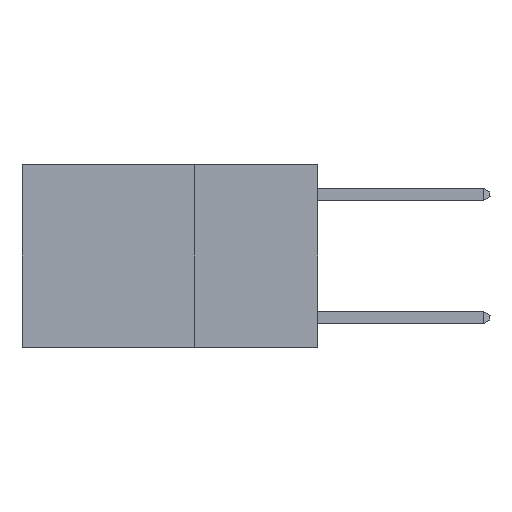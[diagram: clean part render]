
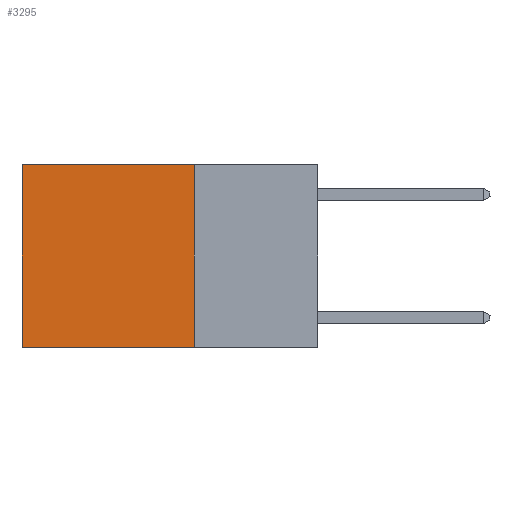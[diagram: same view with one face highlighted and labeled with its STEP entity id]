
A CAD part, left-side view. The second image highlights one B-rep face of the part: STEP entity #3295.
In plain terms, the highlighted planar face has unit normal (-1, 0, 0).
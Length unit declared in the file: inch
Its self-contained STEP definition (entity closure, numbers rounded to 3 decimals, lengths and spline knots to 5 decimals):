
#916 = ORIENTED_EDGE ( 'NONE', *, *, #24766, .T. ) ;
#2970 = VECTOR ( 'NONE', #10923, 39.37008 ) ;
#3295 = ADVANCED_FACE ( 'NONE', ( #18568 ), #12385, .F. ) ;
#3473 = DIRECTION ( 'NONE',  ( 1., 0., 0. ) ) ;
#4056 = DIRECTION ( 'NONE',  ( 0., 0., -1. ) ) ;
#4221 = VERTEX_POINT ( 'NONE', #8551 ) ;
#4352 = VERTEX_POINT ( 'NONE', #13486 ) ;
#6015 = ORIENTED_EDGE ( 'NONE', *, *, #16550, .F. ) ;
#8277 = CARTESIAN_POINT ( 'NONE',  ( 0.2625, 0.6, 0. ) ) ;
#8551 = CARTESIAN_POINT ( 'NONE',  ( 0.2625, 0.6, -0.37 ) ) ;
#8670 = CARTESIAN_POINT ( 'NONE',  ( 0.2625, 0.25, -0.37 ) ) ;
#10423 = LINE ( 'NONE', #16756, #11601 ) ;
#10604 = ORIENTED_EDGE ( 'NONE', *, *, #14463, .T. ) ;
#10695 = VECTOR ( 'NONE', #12228, 39.37008 ) ;
#10923 = DIRECTION ( 'NONE',  ( 0., 1., 0. ) ) ;
#11601 = VECTOR ( 'NONE', #4056, 39.37008 ) ;
#12228 = DIRECTION ( 'NONE',  ( 0., 0., -1. ) ) ;
#12278 = CARTESIAN_POINT ( 'NONE',  ( 0.2625, 0.25, 0. ) ) ;
#12385 = PLANE ( 'NONE',  #26535 ) ;
#12756 = VERTEX_POINT ( 'NONE', #12278 ) ;
#13092 = EDGE_LOOP ( 'NONE', ( #916, #6015, #21237, #10604 ) ) ;
#13486 = CARTESIAN_POINT ( 'NONE',  ( 0.2625, 0.25, -0.37 ) ) ;
#14463 = EDGE_CURVE ( 'NONE', #12756, #21655, #22265, .T. ) ;
#16550 = EDGE_CURVE ( 'NONE', #4352, #4221, #27836, .T. ) ;
#16756 = CARTESIAN_POINT ( 'NONE',  ( 0.2625, 0.25, 0. ) ) ;
#16844 = LINE ( 'NONE', #23070, #10695 ) ;
#17930 = EDGE_CURVE ( 'NONE', #12756, #4352, #10423, .T. ) ;
#18568 = FACE_OUTER_BOUND ( 'NONE', #13092, .T. ) ;
#20975 = DIRECTION ( 'NONE',  ( 0., 0., -1. ) ) ;
#21237 = ORIENTED_EDGE ( 'NONE', *, *, #17930, .F. ) ;
#21655 = VERTEX_POINT ( 'NONE', #8277 ) ;
#22265 = LINE ( 'NONE', #24377, #25045 ) ;
#23070 = CARTESIAN_POINT ( 'NONE',  ( 0.2625, 0.6, 0. ) ) ;
#24377 = CARTESIAN_POINT ( 'NONE',  ( 0.2625, 0.25, 0. ) ) ;
#24766 = EDGE_CURVE ( 'NONE', #21655, #4221, #16844, .T. ) ;
#25045 = VECTOR ( 'NONE', #26616, 39.37008 ) ;
#26535 = AXIS2_PLACEMENT_3D ( 'NONE', #27454, #3473, #20975 ) ;
#26616 = DIRECTION ( 'NONE',  ( 0., 1., 0. ) ) ;
#27454 = CARTESIAN_POINT ( 'NONE',  ( 0.2625, 0.25, 0. ) ) ;
#27836 = LINE ( 'NONE', #8670, #2970 ) ;
